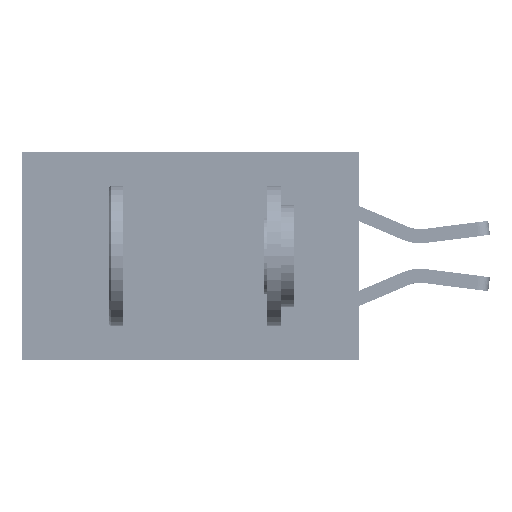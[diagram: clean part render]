
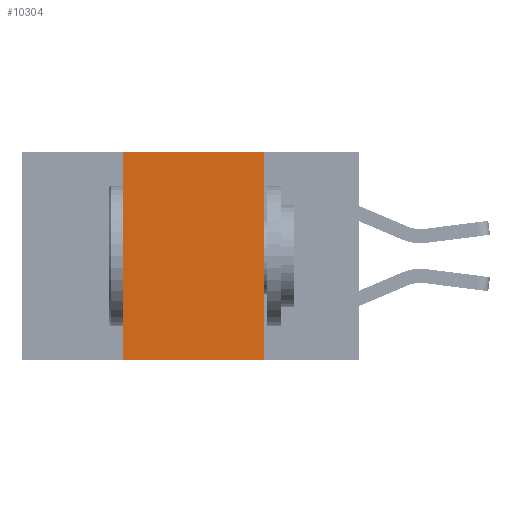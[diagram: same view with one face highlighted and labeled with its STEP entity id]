
A CAD part, left-side view. The second image highlights one B-rep face of the part: STEP entity #10304.
In plain terms, the highlighted planar face has unit normal (-1, 0, 0).
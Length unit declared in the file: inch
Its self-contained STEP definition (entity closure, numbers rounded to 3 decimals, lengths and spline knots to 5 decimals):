
#327 = DIRECTION ( 'NONE',  ( 0., 0., -1. ) ) ;
#556 = CARTESIAN_POINT ( 'NONE',  ( 0., 0.42, 0. ) ) ;
#593 = LINE ( 'NONE', #5431, #30494 ) ;
#852 = CARTESIAN_POINT ( 'NONE',  ( 0., 0.17, -0.37 ) ) ;
#1583 = EDGE_LOOP ( 'NONE', ( #17367, #35750, #28623, #25892 ) ) ;
#3073 = PLANE ( 'NONE',  #30617 ) ;
#4159 = VECTOR ( 'NONE', #5061, 39.37008 ) ;
#5061 = DIRECTION ( 'NONE',  ( 0., 0., 1. ) ) ;
#5431 = CARTESIAN_POINT ( 'NONE',  ( 0., 0.17, 0. ) ) ;
#6014 = EDGE_CURVE ( 'NONE', #18755, #33201, #32041, .T. ) ;
#6307 = DIRECTION ( 'NONE',  ( 1., 0., 0. ) ) ;
#9417 = EDGE_CURVE ( 'NONE', #33201, #24887, #593, .T. ) ;
#9661 = DIRECTION ( 'NONE',  ( 0., -1., 0. ) ) ;
#10304 = ADVANCED_FACE ( 'NONE', ( #14521 ), #3073, .F. ) ;
#11039 = CARTESIAN_POINT ( 'NONE',  ( 0., 0.17, 0. ) ) ;
#13661 = EDGE_CURVE ( 'NONE', #33307, #24887, #30975, .T. ) ;
#14521 = FACE_OUTER_BOUND ( 'NONE', #1583, .T. ) ;
#14774 = CARTESIAN_POINT ( 'NONE',  ( 0., 0.6, -0.37 ) ) ;
#16211 = EDGE_CURVE ( 'NONE', #33307, #18755, #24758, .T. ) ;
#17367 = ORIENTED_EDGE ( 'NONE', *, *, #9417, .F. ) ;
#18755 = VERTEX_POINT ( 'NONE', #556 ) ;
#20415 = CARTESIAN_POINT ( 'NONE',  ( 0., 0.42, -0.37 ) ) ;
#20775 = CARTESIAN_POINT ( 'NONE',  ( 0., 0.6, 0. ) ) ;
#21644 = VECTOR ( 'NONE', #9661, 39.37008 ) ;
#24758 = LINE ( 'NONE', #37830, #4159 ) ;
#24887 = VERTEX_POINT ( 'NONE', #852 ) ;
#25892 = ORIENTED_EDGE ( 'NONE', *, *, #13661, .T. ) ;
#26348 = DIRECTION ( 'NONE',  ( 0., 0., -1. ) ) ;
#28623 = ORIENTED_EDGE ( 'NONE', *, *, #16211, .F. ) ;
#30494 = VECTOR ( 'NONE', #26348, 39.37008 ) ;
#30617 = AXIS2_PLACEMENT_3D ( 'NONE', #20775, #6307, #327 ) ;
#30975 = LINE ( 'NONE', #14774, #21644 ) ;
#31465 = CARTESIAN_POINT ( 'NONE',  ( 0., 0.6, 0. ) ) ;
#32041 = LINE ( 'NONE', #31465, #37151 ) ;
#33201 = VERTEX_POINT ( 'NONE', #11039 ) ;
#33307 = VERTEX_POINT ( 'NONE', #20415 ) ;
#34086 = DIRECTION ( 'NONE',  ( 0., -1., 0. ) ) ;
#35750 = ORIENTED_EDGE ( 'NONE', *, *, #6014, .F. ) ;
#37151 = VECTOR ( 'NONE', #34086, 39.37008 ) ;
#37830 = CARTESIAN_POINT ( 'NONE',  ( 0., 0.42, 0. ) ) ;
